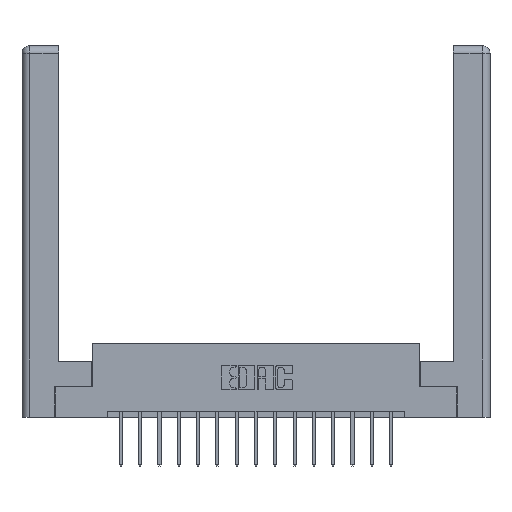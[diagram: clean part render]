
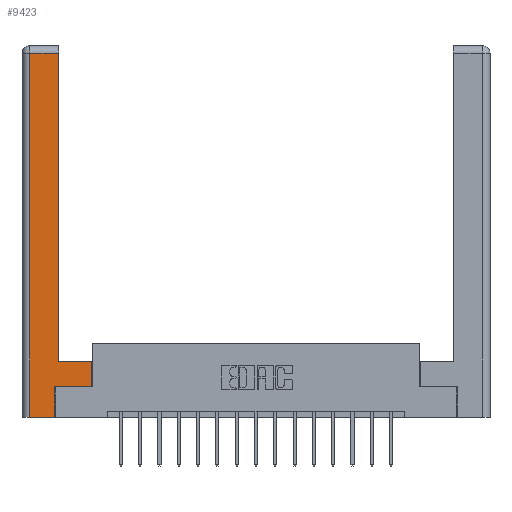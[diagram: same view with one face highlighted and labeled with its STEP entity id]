
A CAD part, top view. The second image highlights one B-rep face of the part: STEP entity #9423.
In plain terms, the highlighted planar face has unit normal (0, 0, 1).
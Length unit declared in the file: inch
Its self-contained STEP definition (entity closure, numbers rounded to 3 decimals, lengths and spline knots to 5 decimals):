
#563 = EDGE_CURVE ( 'NONE', #16067, #12080, #15058, .T. ) ;
#731 = CARTESIAN_POINT ( 'NONE',  ( 0.295, 3., 0. ) ) ;
#920 = VECTOR ( 'NONE', #8293, 39.37008 ) ;
#1474 = VECTOR ( 'NONE', #4642, 39.37008 ) ;
#1816 = VECTOR ( 'NONE', #3859, 39.37008 ) ;
#1988 = VECTOR ( 'NONE', #14941, 39.37008 ) ;
#2154 = CARTESIAN_POINT ( 'NONE',  ( 0.565, 0.45, 0. ) ) ;
#2193 = CARTESIAN_POINT ( 'NONE',  ( 0., 0., 0. ) ) ;
#2282 = DIRECTION ( 'NONE',  ( 0., 1., 0. ) ) ;
#2537 = VECTOR ( 'NONE', #13683, 39.37008 ) ;
#2617 = CARTESIAN_POINT ( 'NONE',  ( 0.565, 0.245, 0. ) ) ;
#2744 = EDGE_LOOP ( 'NONE', ( #13324, #11797, #17031, #14253, #8370, #10585, #8546, #13737 ) ) ;
#2780 = VECTOR ( 'NONE', #14204, 39.37008 ) ;
#3859 = DIRECTION ( 'NONE',  ( 1., 0., 0. ) ) ;
#4488 = VERTEX_POINT ( 'NONE', #7330 ) ;
#4642 = DIRECTION ( 'NONE',  ( 0., 1., 0. ) ) ;
#4883 = FACE_OUTER_BOUND ( 'NONE', #2744, .T. ) ;
#5883 = DIRECTION ( 'NONE',  ( 1., 0., 0. ) ) ;
#6531 = CARTESIAN_POINT ( 'NONE',  ( 0.295, 2.94, 0. ) ) ;
#6842 = LINE ( 'NONE', #731, #1474 ) ;
#7203 = CARTESIAN_POINT ( 'NONE',  ( 0.0615, 0., 0. ) ) ;
#7330 = CARTESIAN_POINT ( 'NONE',  ( 0.265, 0.245, 0. ) ) ;
#7474 = LINE ( 'NONE', #7203, #2780 ) ;
#7649 = CARTESIAN_POINT ( 'NONE',  ( 0.0615, 2.94, 0. ) ) ;
#8293 = DIRECTION ( 'NONE',  ( -1., 0., 0. ) ) ;
#8370 = ORIENTED_EDGE ( 'NONE', *, *, #17494, .T. ) ;
#8546 = ORIENTED_EDGE ( 'NONE', *, *, #563, .T. ) ;
#8847 = VECTOR ( 'NONE', #5883, 39.37008 ) ;
#8998 = PLANE ( 'NONE',  #15547 ) ;
#9084 = CARTESIAN_POINT ( 'NONE',  ( 0.565, 0.45, 0. ) ) ;
#9423 = ADVANCED_FACE ( 'NONE', ( #4883 ), #8998, .F. ) ;
#10182 = LINE ( 'NONE', #12033, #1816 ) ;
#10585 = ORIENTED_EDGE ( 'NONE', *, *, #11564, .T. ) ;
#11030 = LINE ( 'NONE', #11354, #8847 ) ;
#11354 = CARTESIAN_POINT ( 'NONE',  ( 0.265, 0., 0. ) ) ;
#11564 = EDGE_CURVE ( 'NONE', #4488, #16067, #10182, .T. ) ;
#11797 = ORIENTED_EDGE ( 'NONE', *, *, #12168, .T. ) ;
#12033 = CARTESIAN_POINT ( 'NONE',  ( 0.565, 0.245, 0. ) ) ;
#12080 = VERTEX_POINT ( 'NONE', #2154 ) ;
#12168 = EDGE_CURVE ( 'NONE', #15198, #13209, #16294, .T. ) ;
#12475 = VECTOR ( 'NONE', #2282, 39.37008 ) ;
#12602 = CARTESIAN_POINT ( 'NONE',  ( 0.295, 0.45, 0. ) ) ;
#12862 = CARTESIAN_POINT ( 'NONE',  ( 0.265, 0., 0. ) ) ;
#13209 = VERTEX_POINT ( 'NONE', #16851 ) ;
#13324 = ORIENTED_EDGE ( 'NONE', *, *, #14028, .T. ) ;
#13382 = LINE ( 'NONE', #13562, #1988 ) ;
#13445 = VERTEX_POINT ( 'NONE', #14451 ) ;
#13562 = CARTESIAN_POINT ( 'NONE',  ( 0.265, 0.245, 0. ) ) ;
#13683 = DIRECTION ( 'NONE',  ( -1., 0., 0. ) ) ;
#13696 = VERTEX_POINT ( 'NONE', #16469 ) ;
#13737 = ORIENTED_EDGE ( 'NONE', *, *, #17573, .T. ) ;
#13883 = EDGE_CURVE ( 'NONE', #13209, #13696, #7474, .T. ) ;
#14028 = EDGE_CURVE ( 'NONE', #13445, #15198, #6842, .T. ) ;
#14204 = DIRECTION ( 'NONE',  ( 0., -1., 0. ) ) ;
#14253 = ORIENTED_EDGE ( 'NONE', *, *, #16662, .T. ) ;
#14451 = CARTESIAN_POINT ( 'NONE',  ( 0.295, 0.45, 0. ) ) ;
#14568 = DIRECTION ( 'NONE',  ( 0., 0., -1. ) ) ;
#14941 = DIRECTION ( 'NONE',  ( 0., 1., 0. ) ) ;
#15058 = LINE ( 'NONE', #9084, #12475 ) ;
#15198 = VERTEX_POINT ( 'NONE', #6531 ) ;
#15547 = AXIS2_PLACEMENT_3D ( 'NONE', #2193, #14568, #17321 ) ;
#15729 = LINE ( 'NONE', #12602, #920 ) ;
#16067 = VERTEX_POINT ( 'NONE', #2617 ) ;
#16294 = LINE ( 'NONE', #7649, #2537 ) ;
#16469 = CARTESIAN_POINT ( 'NONE',  ( 0.0615, 0., 0. ) ) ;
#16662 = EDGE_CURVE ( 'NONE', #13696, #17253, #11030, .T. ) ;
#16851 = CARTESIAN_POINT ( 'NONE',  ( 0.0615, 2.94, 0. ) ) ;
#17031 = ORIENTED_EDGE ( 'NONE', *, *, #13883, .T. ) ;
#17253 = VERTEX_POINT ( 'NONE', #12862 ) ;
#17321 = DIRECTION ( 'NONE',  ( -1., 0., 0. ) ) ;
#17494 = EDGE_CURVE ( 'NONE', #17253, #4488, #13382, .T. ) ;
#17573 = EDGE_CURVE ( 'NONE', #12080, #13445, #15729, .T. ) ;
